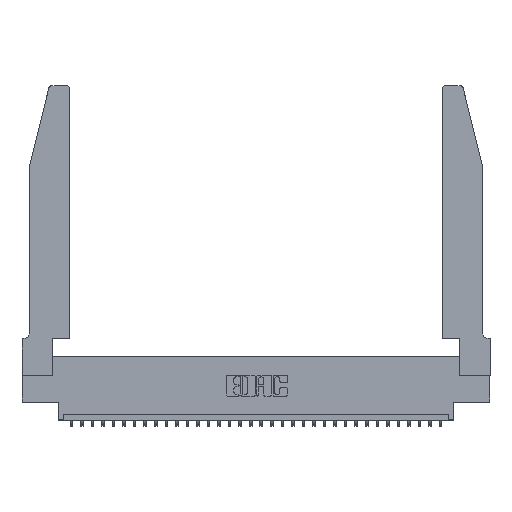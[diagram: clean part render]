
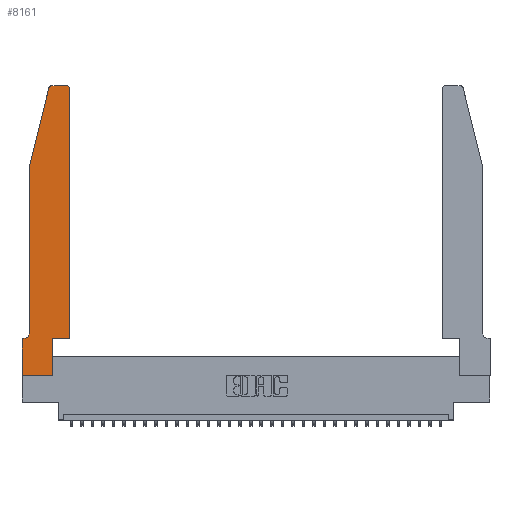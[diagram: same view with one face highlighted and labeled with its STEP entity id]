
A CAD part, top view. The second image highlights one B-rep face of the part: STEP entity #8161.
In plain terms, the highlighted planar face has unit normal (0, 0, 1).
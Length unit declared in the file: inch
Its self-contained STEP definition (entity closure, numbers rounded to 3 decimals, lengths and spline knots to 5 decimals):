
#615 = CARTESIAN_POINT ( 'NONE',  ( 0.284, 2.75, 0.37 ) ) ;
#642 = DIRECTION ( 'NONE',  ( 0., 1., 0. ) ) ;
#649 = ORIENTED_EDGE ( 'NONE', *, *, #27300, .T. ) ;
#1021 = VERTEX_POINT ( 'NONE', #2833 ) ;
#1659 = AXIS2_PLACEMENT_3D ( 'NONE', #19644, #11964, #22220 ) ;
#1676 = EDGE_CURVE ( 'NONE', #32214, #14926, #27164, .T. ) ;
#2082 = CARTESIAN_POINT ( 'NONE',  ( 0.0755, 2., 0.37 ) ) ;
#2087 = ORIENTED_EDGE ( 'NONE', *, *, #31841, .T. ) ;
#2564 = CIRCLE ( 'NONE', #2742, 0.03 ) ;
#2634 = LINE ( 'NONE', #3957, #27702 ) ;
#2650 = CIRCLE ( 'NONE', #1659, 0.03 ) ;
#2742 = AXIS2_PLACEMENT_3D ( 'NONE', #15586, #18126, #30681 ) ;
#2833 = CARTESIAN_POINT ( 'NONE',  ( 0.2865, 0.35, 0.37 ) ) ;
#3625 = EDGE_CURVE ( 'NONE', #30035, #32157, #2564, .T. ) ;
#3957 = CARTESIAN_POINT ( 'NONE',  ( 0., 0., 0.37 ) ) ;
#4271 = EDGE_CURVE ( 'NONE', #28949, #10635, #29149, .T. ) ;
#4430 = CARTESIAN_POINT ( 'NONE',  ( 0.4505, 0.35, 0.37 ) ) ;
#5002 = DIRECTION ( 'NONE',  ( 0., 0., 1. ) ) ;
#5741 = CARTESIAN_POINT ( 'NONE',  ( 0.2865, 0.35, 0.37 ) ) ;
#5839 = CARTESIAN_POINT ( 'NONE',  ( 0.4505, 0.35, 0.37 ) ) ;
#5954 = DIRECTION ( 'NONE',  ( -0.239, -0.971, 0. ) ) ;
#6091 = CARTESIAN_POINT ( 'NONE',  ( 0.4505, 2.72, 0.37 ) ) ;
#6795 = CARTESIAN_POINT ( 'NONE',  ( 0.0055, 0.42, 0.37 ) ) ;
#6853 = VERTEX_POINT ( 'NONE', #2082 ) ;
#7100 = ORIENTED_EDGE ( 'NONE', *, *, #1676, .T. ) ;
#7358 = VERTEX_POINT ( 'NONE', #27468 ) ;
#7369 = DIRECTION ( 'NONE',  ( 1., 0., 0. ) ) ;
#8157 = EDGE_LOOP ( 'NONE', ( #28898, #30837, #21388, #20596, #15499, #12422, #21530, #7100, #19554, #21779, #649, #2087 ) ) ;
#8161 = ADVANCED_FACE ( 'NONE', ( #24585 ), #32642, .T. ) ;
#8284 = CARTESIAN_POINT ( 'NONE',  ( 0., 0., 0.37 ) ) ;
#8305 = VECTOR ( 'NONE', #7369, 39.37008 ) ;
#8796 = CARTESIAN_POINT ( 'NONE',  ( 0.2865, 0., 0.37 ) ) ;
#9473 = LINE ( 'NONE', #27516, #8305 ) ;
#9645 = DIRECTION ( 'NONE',  ( 1., 0., 0. ) ) ;
#9804 = CARTESIAN_POINT ( 'NONE',  ( 0.0755, 0.42, 0.37 ) ) ;
#10338 = CARTESIAN_POINT ( 'NONE',  ( 0.0055, 0.35, 0.37 ) ) ;
#10635 = VERTEX_POINT ( 'NONE', #10338 ) ;
#10868 = VECTOR ( 'NONE', #24421, 39.37008 ) ;
#11196 = CARTESIAN_POINT ( 'NONE',  ( 0., 0., 0.37 ) ) ;
#11964 = DIRECTION ( 'NONE',  ( 0., 0., 1. ) ) ;
#12422 = ORIENTED_EDGE ( 'NONE', *, *, #17524, .T. ) ;
#12521 = CARTESIAN_POINT ( 'NONE',  ( 0.2605, 2.75, 0.37 ) ) ;
#14374 = VECTOR ( 'NONE', #5954, 39.37008 ) ;
#14829 = EDGE_CURVE ( 'NONE', #6853, #28949, #27224, .T. ) ;
#14890 = VECTOR ( 'NONE', #22816, 39.37008 ) ;
#14926 = VERTEX_POINT ( 'NONE', #8796 ) ;
#15115 = EDGE_CURVE ( 'NONE', #1021, #25763, #9473, .T. ) ;
#15499 = ORIENTED_EDGE ( 'NONE', *, *, #4271, .T. ) ;
#15586 = CARTESIAN_POINT ( 'NONE',  ( 0.284, 2.72, 0.37 ) ) ;
#15710 = LINE ( 'NONE', #27699, #14890 ) ;
#15989 = LINE ( 'NONE', #18618, #14374 ) ;
#16235 = DIRECTION ( 'NONE',  ( 1., 0., 0. ) ) ;
#16677 = AXIS2_PLACEMENT_3D ( 'NONE', #27477, #5002, #9645 ) ;
#16792 = EDGE_CURVE ( 'NONE', #7358, #32214, #2634, .T. ) ;
#17221 = VECTOR ( 'NONE', #30281, 39.37008 ) ;
#17524 = EDGE_CURVE ( 'NONE', #10635, #7358, #15710, .T. ) ;
#18126 = DIRECTION ( 'NONE',  ( 0., 0., 1. ) ) ;
#18618 = CARTESIAN_POINT ( 'NONE',  ( 0.0755, 2., 0.37 ) ) ;
#18789 = LINE ( 'NONE', #12521, #17221 ) ;
#18834 = VECTOR ( 'NONE', #642, 39.37008 ) ;
#19554 = ORIENTED_EDGE ( 'NONE', *, *, #22984, .T. ) ;
#19597 = EDGE_CURVE ( 'NONE', #29725, #30035, #18789, .T. ) ;
#19644 = CARTESIAN_POINT ( 'NONE',  ( 0.4205, 2.72, 0.37 ) ) ;
#19836 = DIRECTION ( 'NONE',  ( 0., -1., 0. ) ) ;
#20596 = ORIENTED_EDGE ( 'NONE', *, *, #14829, .T. ) ;
#20997 = CARTESIAN_POINT ( 'NONE',  ( 0.25487, 2.72718, 0.37 ) ) ;
#21249 = LINE ( 'NONE', #5839, #18834 ) ;
#21388 = ORIENTED_EDGE ( 'NONE', *, *, #29432, .T. ) ;
#21530 = ORIENTED_EDGE ( 'NONE', *, *, #16792, .T. ) ;
#21733 = AXIS2_PLACEMENT_3D ( 'NONE', #6795, #29482, #24726 ) ;
#21779 = ORIENTED_EDGE ( 'NONE', *, *, #15115, .T. ) ;
#22174 = CARTESIAN_POINT ( 'NONE',  ( 0.4205, 2.75, 0.37 ) ) ;
#22220 = DIRECTION ( 'NONE',  ( 1., 0., 0. ) ) ;
#22816 = DIRECTION ( 'NONE',  ( -1., 0., 0. ) ) ;
#22984 = EDGE_CURVE ( 'NONE', #14926, #1021, #28708, .T. ) ;
#23554 = VECTOR ( 'NONE', #25754, 39.37008 ) ;
#24098 = CARTESIAN_POINT ( 'NONE',  ( 0.0755, 2., 0.37 ) ) ;
#24421 = DIRECTION ( 'NONE',  ( 0., -1., 0. ) ) ;
#24585 = FACE_OUTER_BOUND ( 'NONE', #8157, .T. ) ;
#24726 = DIRECTION ( 'NONE',  ( -1., 0., 0. ) ) ;
#25754 = DIRECTION ( 'NONE',  ( 0., 1., 0. ) ) ;
#25763 = VERTEX_POINT ( 'NONE', #4430 ) ;
#27164 = LINE ( 'NONE', #11196, #32288 ) ;
#27224 = LINE ( 'NONE', #24098, #10868 ) ;
#27300 = EDGE_CURVE ( 'NONE', #25763, #31683, #21249, .T. ) ;
#27468 = CARTESIAN_POINT ( 'NONE',  ( 0., 0.35, 0.37 ) ) ;
#27477 = CARTESIAN_POINT ( 'NONE',  ( 0., 0.35, 0.37 ) ) ;
#27516 = CARTESIAN_POINT ( 'NONE',  ( 0.4505, 0.35, 0.37 ) ) ;
#27699 = CARTESIAN_POINT ( 'NONE',  ( 0.0755, 0.35, 0.37 ) ) ;
#27702 = VECTOR ( 'NONE', #19836, 39.37008 ) ;
#28708 = LINE ( 'NONE', #5741, #23554 ) ;
#28898 = ORIENTED_EDGE ( 'NONE', *, *, #19597, .T. ) ;
#28949 = VERTEX_POINT ( 'NONE', #9804 ) ;
#29149 = CIRCLE ( 'NONE', #21733, 0.07 ) ;
#29432 = EDGE_CURVE ( 'NONE', #32157, #6853, #15989, .T. ) ;
#29482 = DIRECTION ( 'NONE',  ( 0., 0., -1. ) ) ;
#29725 = VERTEX_POINT ( 'NONE', #22174 ) ;
#30035 = VERTEX_POINT ( 'NONE', #615 ) ;
#30281 = DIRECTION ( 'NONE',  ( -1., 0., 0. ) ) ;
#30681 = DIRECTION ( 'NONE',  ( 1., 0., 0. ) ) ;
#30837 = ORIENTED_EDGE ( 'NONE', *, *, #3625, .T. ) ;
#31683 = VERTEX_POINT ( 'NONE', #6091 ) ;
#31841 = EDGE_CURVE ( 'NONE', #31683, #29725, #2650, .T. ) ;
#32157 = VERTEX_POINT ( 'NONE', #20997 ) ;
#32214 = VERTEX_POINT ( 'NONE', #8284 ) ;
#32288 = VECTOR ( 'NONE', #16235, 39.37008 ) ;
#32642 = PLANE ( 'NONE',  #16677 ) ;
